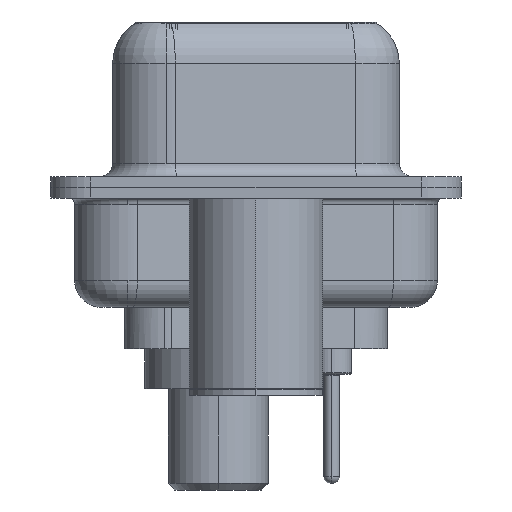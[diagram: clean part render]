
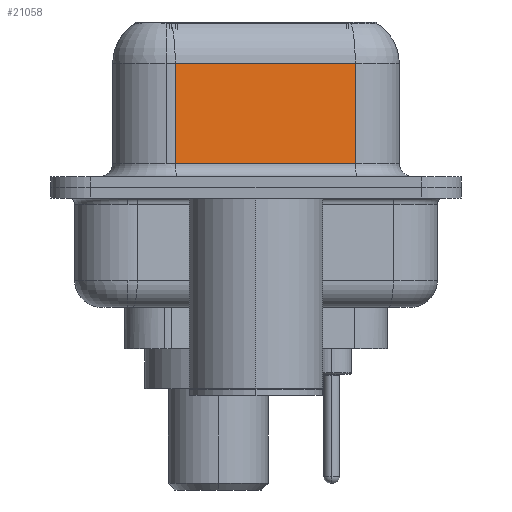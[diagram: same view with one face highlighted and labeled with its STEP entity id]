
A CAD part, left-side view. The second image highlights one B-rep face of the part: STEP entity #21058.
In plain terms, the highlighted planar face has unit normal (-0.985, -0.174, 0).
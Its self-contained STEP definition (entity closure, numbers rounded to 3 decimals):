
#668 = VERTEX_POINT ( 'NONE', #15801 ) ;
#1040 = DIRECTION ( 'NONE',  ( 0.985, 0.174, 0. ) ) ;
#1610 = VERTEX_POINT ( 'NONE', #30685 ) ;
#2651 = EDGE_LOOP ( 'NONE', ( #26335, #32568, #19698, #15017 ) ) ;
#3112 = AXIS2_PLACEMENT_3D ( 'NONE', #16855, #1040, #11506 ) ;
#4595 = LINE ( 'NONE', #19283, #25996 ) ;
#5062 = LINE ( 'NONE', #28070, #33160 ) ;
#6435 = EDGE_CURVE ( 'NONE', #668, #30984, #5062, .T. ) ;
#6696 = DIRECTION ( 'NONE',  ( 0., 0., -1. ) ) ;
#7933 = FACE_OUTER_BOUND ( 'NONE', #2651, .T. ) ;
#7985 = CARTESIAN_POINT ( 'NONE',  ( 5.621, -3.722, 0.9 ) ) ;
#10073 = DIRECTION ( 'NONE',  ( 0.174, -0.985, 0. ) ) ;
#10649 = EDGE_CURVE ( 'NONE', #24848, #1610, #4595, .T. ) ;
#10872 = LINE ( 'NONE', #7985, #24296 ) ;
#11506 = DIRECTION ( 'NONE',  ( -0.174, 0.985, 0. ) ) ;
#15017 = ORIENTED_EDGE ( 'NONE', *, *, #25763, .T. ) ;
#15046 = VECTOR ( 'NONE', #32089, 1000. ) ;
#15801 = CARTESIAN_POINT ( 'NONE',  ( 5.621, -3.722, 4.65 ) ) ;
#16855 = CARTESIAN_POINT ( 'NONE',  ( 5.621, -3.722, 6.4 ) ) ;
#18392 = LINE ( 'NONE', #21492, #15046 ) ;
#19283 = CARTESIAN_POINT ( 'NONE',  ( 4.43, 3.028, 6.4 ) ) ;
#19698 = ORIENTED_EDGE ( 'NONE', *, *, #10649, .T. ) ;
#21058 = ADVANCED_FACE ( 'NONE', ( #7933 ), #33352, .F. ) ;
#21492 = CARTESIAN_POINT ( 'NONE',  ( 5.621, -3.722, 4.65 ) ) ;
#22795 = CARTESIAN_POINT ( 'NONE',  ( 4.43, 3.028, 4.65 ) ) ;
#24296 = VECTOR ( 'NONE', #10073, 1000. ) ;
#24362 = DIRECTION ( 'NONE',  ( 0., 0., -1. ) ) ;
#24848 = VERTEX_POINT ( 'NONE', #22795 ) ;
#25134 = EDGE_CURVE ( 'NONE', #668, #24848, #18392, .T. ) ;
#25763 = EDGE_CURVE ( 'NONE', #1610, #30984, #10872, .T. ) ;
#25895 = CARTESIAN_POINT ( 'NONE',  ( 5.621, -3.722, 0.9 ) ) ;
#25996 = VECTOR ( 'NONE', #24362, 1000. ) ;
#26335 = ORIENTED_EDGE ( 'NONE', *, *, #6435, .F. ) ;
#28070 = CARTESIAN_POINT ( 'NONE',  ( 5.621, -3.722, 6.4 ) ) ;
#30685 = CARTESIAN_POINT ( 'NONE',  ( 4.43, 3.028, 0.9 ) ) ;
#30984 = VERTEX_POINT ( 'NONE', #25895 ) ;
#32089 = DIRECTION ( 'NONE',  ( -0.174, 0.985, 0. ) ) ;
#32568 = ORIENTED_EDGE ( 'NONE', *, *, #25134, .T. ) ;
#33160 = VECTOR ( 'NONE', #6696, 1000. ) ;
#33352 = PLANE ( 'NONE',  #3112 ) ;
